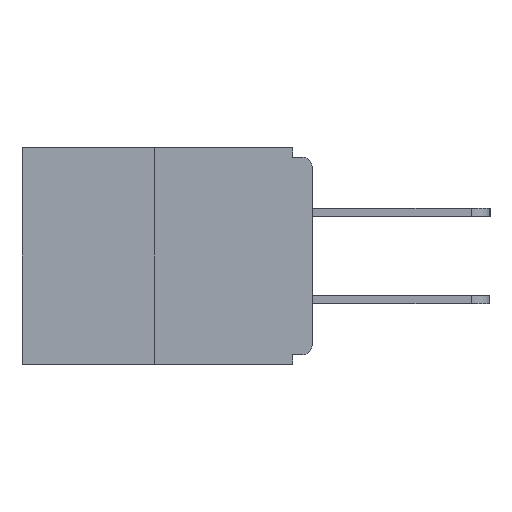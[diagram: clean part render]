
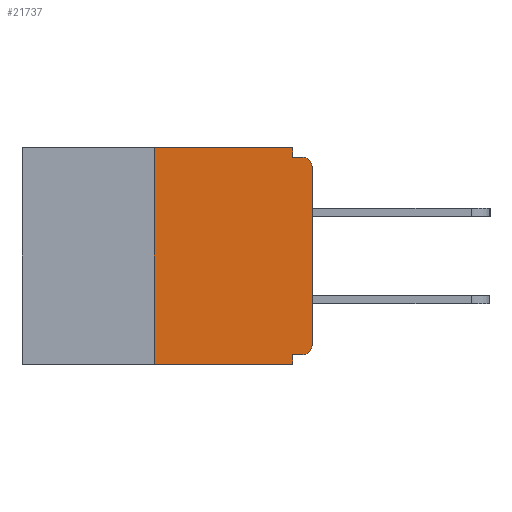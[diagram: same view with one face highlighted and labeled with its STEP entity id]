
A CAD part, left-side view. The second image highlights one B-rep face of the part: STEP entity #21737.
In plain terms, the highlighted planar face has unit normal (-1, 0, 0).
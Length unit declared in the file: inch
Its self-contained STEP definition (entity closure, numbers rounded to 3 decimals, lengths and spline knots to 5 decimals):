
#421 = ORIENTED_EDGE ( 'NONE', *, *, #12014, .T. ) ;
#474 = CARTESIAN_POINT ( 'NONE',  ( 0., 0.015, -0.015 ) ) ;
#510 = VERTEX_POINT ( 'NONE', #18771 ) ;
#539 = LINE ( 'NONE', #11088, #10516 ) ;
#587 = CIRCLE ( 'NONE', #8163, 0.015 ) ;
#608 = CARTESIAN_POINT ( 'NONE',  ( 0., 0., 0. ) ) ;
#1015 = EDGE_CURVE ( 'NONE', #18262, #19291, #2116, .T. ) ;
#2116 = CIRCLE ( 'NONE', #2474, 0.015 ) ;
#2474 = AXIS2_PLACEMENT_3D ( 'NONE', #19123, #2960, #16473 ) ;
#2906 = CARTESIAN_POINT ( 'NONE',  ( 0., 0., -0.03 ) ) ;
#2960 = DIRECTION ( 'NONE',  ( -1., 0., 0. ) ) ;
#3198 = VERTEX_POINT ( 'NONE', #3865 ) ;
#3704 = CARTESIAN_POINT ( 'NONE',  ( 0., 0.031, -0.343 ) ) ;
#3856 = VERTEX_POINT ( 'NONE', #21741 ) ;
#3865 = CARTESIAN_POINT ( 'NONE',  ( 0., 0.031, -0.328 ) ) ;
#4197 = DIRECTION ( 'NONE',  ( 0., 0., 1. ) ) ;
#4300 = DIRECTION ( 'NONE',  ( 0., 0., -1. ) ) ;
#4451 = DIRECTION ( 'NONE',  ( 0., 0., -1. ) ) ;
#4729 = CARTESIAN_POINT ( 'NONE',  ( 0., 0.25, 0. ) ) ;
#4730 = EDGE_LOOP ( 'NONE', ( #17123, #17427, #16593, #18157, #11784, #13707, #421, #14195, #8034, #5027 ) ) ;
#5027 = ORIENTED_EDGE ( 'NONE', *, *, #18365, .F. ) ;
#6045 = DIRECTION ( 'NONE',  ( 0., 1., 0. ) ) ;
#6196 = EDGE_CURVE ( 'NONE', #16842, #17236, #6332, .T. ) ;
#6322 = CARTESIAN_POINT ( 'NONE',  ( 0., 0.25, -0.343 ) ) ;
#6332 = LINE ( 'NONE', #20387, #13240 ) ;
#6457 = CARTESIAN_POINT ( 'NONE',  ( 0., 0.46, 0. ) ) ;
#6575 = VECTOR ( 'NONE', #14119, 39.37008 ) ;
#6842 = CARTESIAN_POINT ( 'NONE',  ( 0., 0.031, 0. ) ) ;
#7331 = CARTESIAN_POINT ( 'NONE',  ( 0., 0.015, -0.03 ) ) ;
#7469 = DIRECTION ( 'NONE',  ( 0., -1., 0. ) ) ;
#7495 = LINE ( 'NONE', #14949, #12427 ) ;
#7936 = LINE ( 'NONE', #6457, #21434 ) ;
#8034 = ORIENTED_EDGE ( 'NONE', *, *, #11299, .F. ) ;
#8163 = AXIS2_PLACEMENT_3D ( 'NONE', #7331, #11403, #4300 ) ;
#8641 = DIRECTION ( 'NONE',  ( 0., 0., -1. ) ) ;
#8881 = CARTESIAN_POINT ( 'NONE',  ( 0., 0., -0.313 ) ) ;
#9385 = EDGE_CURVE ( 'NONE', #16842, #20412, #21890, .T. ) ;
#9682 = DIRECTION ( 'NONE',  ( 1., 0., 0. ) ) ;
#9867 = DIRECTION ( 'NONE',  ( 0., -1., 0. ) ) ;
#10030 = DIRECTION ( 'NONE',  ( 0., 0., 1. ) ) ;
#10139 = VERTEX_POINT ( 'NONE', #2906 ) ;
#10516 = VECTOR ( 'NONE', #7469, 39.37008 ) ;
#10843 = CARTESIAN_POINT ( 'NONE',  ( 0., 0.25, 0. ) ) ;
#11088 = CARTESIAN_POINT ( 'NONE',  ( 0., 0., -0.015 ) ) ;
#11299 = EDGE_CURVE ( 'NONE', #510, #11323, #539, .T. ) ;
#11323 = VERTEX_POINT ( 'NONE', #474 ) ;
#11392 = EDGE_CURVE ( 'NONE', #18262, #3198, #7495, .T. ) ;
#11403 = DIRECTION ( 'NONE',  ( -1., 0., 0. ) ) ;
#11784 = ORIENTED_EDGE ( 'NONE', *, *, #11392, .F. ) ;
#12011 = FACE_OUTER_BOUND ( 'NONE', #4730, .T. ) ;
#12014 = EDGE_CURVE ( 'NONE', #19291, #10139, #20349, .T. ) ;
#12320 = CARTESIAN_POINT ( 'NONE',  ( 0., 0.015, -0.328 ) ) ;
#12427 = VECTOR ( 'NONE', #6045, 39.37008 ) ;
#13240 = VECTOR ( 'NONE', #16854, 39.37008 ) ;
#13657 = EDGE_CURVE ( 'NONE', #20412, #3856, #7936, .T. ) ;
#13707 = ORIENTED_EDGE ( 'NONE', *, *, #1015, .T. ) ;
#14119 = DIRECTION ( 'NONE',  ( 0., 0., -1. ) ) ;
#14195 = ORIENTED_EDGE ( 'NONE', *, *, #19858, .T. ) ;
#14949 = CARTESIAN_POINT ( 'NONE',  ( 0., 0., -0.328 ) ) ;
#14959 = CARTESIAN_POINT ( 'NONE',  ( 0., 0.46, 0. ) ) ;
#15690 = VECTOR ( 'NONE', #4197, 39.37008 ) ;
#15818 = EDGE_CURVE ( 'NONE', #3198, #17236, #22544, .T. ) ;
#16473 = DIRECTION ( 'NONE',  ( 0., 0., -1. ) ) ;
#16593 = ORIENTED_EDGE ( 'NONE', *, *, #6196, .T. ) ;
#16842 = VERTEX_POINT ( 'NONE', #6322 ) ;
#16854 = DIRECTION ( 'NONE',  ( 0., -1., 0. ) ) ;
#17123 = ORIENTED_EDGE ( 'NONE', *, *, #13657, .F. ) ;
#17236 = VERTEX_POINT ( 'NONE', #3704 ) ;
#17427 = ORIENTED_EDGE ( 'NONE', *, *, #9385, .F. ) ;
#18042 = AXIS2_PLACEMENT_3D ( 'NONE', #14959, #9682, #4451 ) ;
#18157 = ORIENTED_EDGE ( 'NONE', *, *, #15818, .F. ) ;
#18262 = VERTEX_POINT ( 'NONE', #12320 ) ;
#18365 = EDGE_CURVE ( 'NONE', #3856, #510, #19110, .T. ) ;
#18771 = CARTESIAN_POINT ( 'NONE',  ( 0., 0.031, -0.015 ) ) ;
#18791 = PLANE ( 'NONE',  #18042 ) ;
#19110 = LINE ( 'NONE', #6842, #22179 ) ;
#19123 = CARTESIAN_POINT ( 'NONE',  ( 0., 0.015, -0.313 ) ) ;
#19291 = VERTEX_POINT ( 'NONE', #8881 ) ;
#19858 = EDGE_CURVE ( 'NONE', #10139, #11323, #587, .T. ) ;
#20221 = VECTOR ( 'NONE', #10030, 39.37008 ) ;
#20349 = LINE ( 'NONE', #608, #15690 ) ;
#20387 = CARTESIAN_POINT ( 'NONE',  ( 0., 0.46, -0.343 ) ) ;
#20412 = VERTEX_POINT ( 'NONE', #10843 ) ;
#21133 = CARTESIAN_POINT ( 'NONE',  ( 0., 0.031, -0.343 ) ) ;
#21434 = VECTOR ( 'NONE', #9867, 39.37008 ) ;
#21737 = ADVANCED_FACE ( 'NONE', ( #12011 ), #18791, .F. ) ;
#21741 = CARTESIAN_POINT ( 'NONE',  ( 0., 0.031, 0. ) ) ;
#21890 = LINE ( 'NONE', #4729, #20221 ) ;
#22179 = VECTOR ( 'NONE', #8641, 39.37008 ) ;
#22544 = LINE ( 'NONE', #21133, #6575 ) ;
